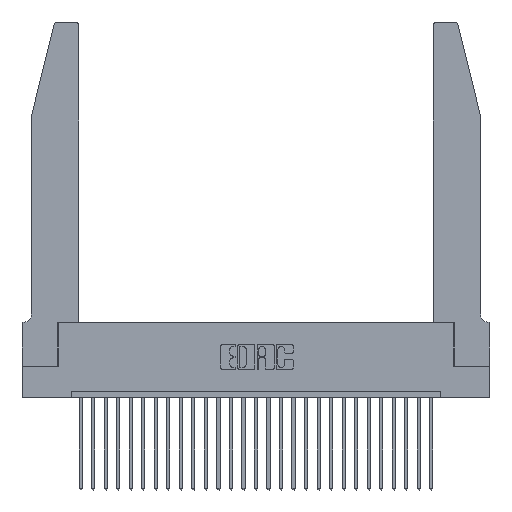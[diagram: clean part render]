
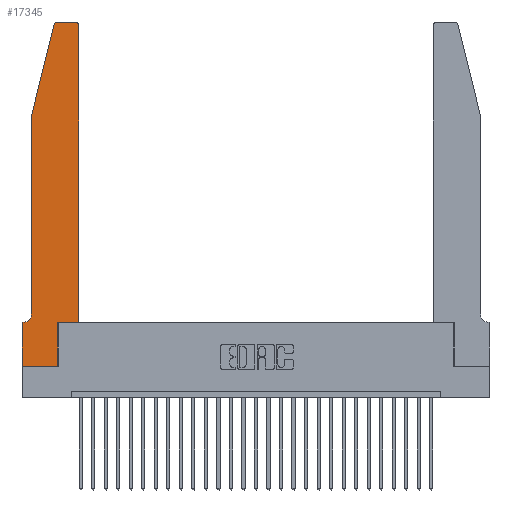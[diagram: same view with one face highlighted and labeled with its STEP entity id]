
A CAD part, top view. The second image highlights one B-rep face of the part: STEP entity #17345.
In plain terms, the highlighted planar face has unit normal (0, 0, 1).
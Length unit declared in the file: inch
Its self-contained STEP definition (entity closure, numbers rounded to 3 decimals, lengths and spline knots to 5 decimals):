
#904 = ORIENTED_EDGE ( 'NONE', *, *, #7573, .T. ) ;
#1580 = EDGE_CURVE ( 'NONE', #14980, #19679, #10628, .T. ) ;
#1957 = CARTESIAN_POINT ( 'NONE',  ( 0.284, 2.72, 0.37 ) ) ;
#2229 = LINE ( 'NONE', #5187, #10463 ) ;
#2458 = CARTESIAN_POINT ( 'NONE',  ( 0.25487, 2.72718, 0.37 ) ) ;
#2658 = CARTESIAN_POINT ( 'NONE',  ( 0., 0., 0.37 ) ) ;
#2712 = CARTESIAN_POINT ( 'NONE',  ( 0.4505, 0.35, 0.37 ) ) ;
#2842 = VERTEX_POINT ( 'NONE', #21856 ) ;
#3408 = ORIENTED_EDGE ( 'NONE', *, *, #24890, .T. ) ;
#3573 = EDGE_CURVE ( 'NONE', #14192, #27895, #18481, .T. ) ;
#3692 = ORIENTED_EDGE ( 'NONE', *, *, #3573, .T. ) ;
#4606 = VERTEX_POINT ( 'NONE', #22567 ) ;
#4884 = CIRCLE ( 'NONE', #19451, 0.07 ) ;
#5000 = ORIENTED_EDGE ( 'NONE', *, *, #16913, .T. ) ;
#5187 = CARTESIAN_POINT ( 'NONE',  ( 0.0755, 0.35, 0.37 ) ) ;
#5272 = VERTEX_POINT ( 'NONE', #11952 ) ;
#5293 = DIRECTION ( 'NONE',  ( -1., 0., 0. ) ) ;
#5399 = VERTEX_POINT ( 'NONE', #17111 ) ;
#5493 = CIRCLE ( 'NONE', #21747, 0.03 ) ;
#5974 = ORIENTED_EDGE ( 'NONE', *, *, #8012, .T. ) ;
#6187 = LINE ( 'NONE', #2658, #23042 ) ;
#6262 = DIRECTION ( 'NONE',  ( 0., 0., 1. ) ) ;
#6360 = AXIS2_PLACEMENT_3D ( 'NONE', #7596, #13937, #27242 ) ;
#6550 = ORIENTED_EDGE ( 'NONE', *, *, #9321, .T. ) ;
#6581 = EDGE_CURVE ( 'NONE', #13716, #5272, #2229, .T. ) ;
#6804 = CARTESIAN_POINT ( 'NONE',  ( 0.4505, 2.72, 0.37 ) ) ;
#7573 = EDGE_CURVE ( 'NONE', #7686, #4606, #26142, .T. ) ;
#7596 = CARTESIAN_POINT ( 'NONE',  ( 0., 0.35, 0.37 ) ) ;
#7686 = VERTEX_POINT ( 'NONE', #14139 ) ;
#8012 = EDGE_CURVE ( 'NONE', #4606, #14192, #25118, .T. ) ;
#8188 = CARTESIAN_POINT ( 'NONE',  ( 0.0755, 2., 0.37 ) ) ;
#8631 = ORIENTED_EDGE ( 'NONE', *, *, #14116, .T. ) ;
#8788 = CARTESIAN_POINT ( 'NONE',  ( 0.4205, 2.75, 0.37 ) ) ;
#9013 = VECTOR ( 'NONE', #11927, 39.37008 ) ;
#9321 = EDGE_CURVE ( 'NONE', #5399, #13716, #4884, .T. ) ;
#10112 = CARTESIAN_POINT ( 'NONE',  ( 0.2865, 0.35, 0.37 ) ) ;
#10231 = VECTOR ( 'NONE', #22392, 39.37008 ) ;
#10463 = VECTOR ( 'NONE', #5293, 39.37008 ) ;
#10628 = LINE ( 'NONE', #15338, #18875 ) ;
#11100 = DIRECTION ( 'NONE',  ( -0.239, -0.971, 0. ) ) ;
#11371 = CARTESIAN_POINT ( 'NONE',  ( 0.284, 2.75, 0.37 ) ) ;
#11375 = DIRECTION ( 'NONE',  ( 0., -1., 0. ) ) ;
#11927 = DIRECTION ( 'NONE',  ( -1., 0., 0. ) ) ;
#11952 = CARTESIAN_POINT ( 'NONE',  ( 0., 0.35, 0.37 ) ) ;
#12058 = DIRECTION ( 'NONE',  ( 0., 0., 1. ) ) ;
#12329 = DIRECTION ( 'NONE',  ( 0., 0., -1. ) ) ;
#12431 = LINE ( 'NONE', #19485, #21072 ) ;
#12522 = ORIENTED_EDGE ( 'NONE', *, *, #25599, .T. ) ;
#12996 = DIRECTION ( 'NONE',  ( 1., 0., 0. ) ) ;
#13116 = CARTESIAN_POINT ( 'NONE',  ( 0.0055, 0.35, 0.37 ) ) ;
#13120 = VECTOR ( 'NONE', #12996, 39.37008 ) ;
#13716 = VERTEX_POINT ( 'NONE', #13116 ) ;
#13937 = DIRECTION ( 'NONE',  ( 0., 0., 1. ) ) ;
#14116 = EDGE_CURVE ( 'NONE', #2842, #7686, #28347, .T. ) ;
#14139 = CARTESIAN_POINT ( 'NONE',  ( 0.2865, 0., 0.37 ) ) ;
#14192 = VERTEX_POINT ( 'NONE', #26556 ) ;
#14232 = CIRCLE ( 'NONE', #27106, 0.03 ) ;
#14272 = DIRECTION ( 'NONE',  ( 1., 0., 0. ) ) ;
#14494 = EDGE_LOOP ( 'NONE', ( #23399, #27559, #21449, #3408, #6550, #26379, #12522, #8631, #904, #5974, #3692, #5000 ) ) ;
#14980 = VERTEX_POINT ( 'NONE', #2458 ) ;
#15338 = CARTESIAN_POINT ( 'NONE',  ( 0.0755, 2., 0.37 ) ) ;
#15766 = CARTESIAN_POINT ( 'NONE',  ( 0., 0., 0.37 ) ) ;
#16856 = CARTESIAN_POINT ( 'NONE',  ( 0.4505, 0.35, 0.37 ) ) ;
#16913 = EDGE_CURVE ( 'NONE', #27895, #18076, #14232, .T. ) ;
#17111 = CARTESIAN_POINT ( 'NONE',  ( 0.0755, 0.42, 0.37 ) ) ;
#17345 = ADVANCED_FACE ( 'NONE', ( #18370 ), #18886, .T. ) ;
#17413 = VECTOR ( 'NONE', #26551, 39.37008 ) ;
#17518 = DIRECTION ( 'NONE',  ( 1., 0., 0. ) ) ;
#18076 = VERTEX_POINT ( 'NONE', #8788 ) ;
#18370 = FACE_OUTER_BOUND ( 'NONE', #14494, .T. ) ;
#18481 = LINE ( 'NONE', #2712, #17413 ) ;
#18562 = VERTEX_POINT ( 'NONE', #11371 ) ;
#18875 = VECTOR ( 'NONE', #11100, 39.37008 ) ;
#18886 = PLANE ( 'NONE',  #6360 ) ;
#19293 = EDGE_CURVE ( 'NONE', #18076, #18562, #27182, .T. ) ;
#19451 = AXIS2_PLACEMENT_3D ( 'NONE', #22994, #12329, #27623 ) ;
#19485 = CARTESIAN_POINT ( 'NONE',  ( 0.0755, 2., 0.37 ) ) ;
#19679 = VERTEX_POINT ( 'NONE', #8188 ) ;
#21072 = VECTOR ( 'NONE', #26139, 39.37008 ) ;
#21449 = ORIENTED_EDGE ( 'NONE', *, *, #1580, .T. ) ;
#21735 = VECTOR ( 'NONE', #25257, 39.37008 ) ;
#21747 = AXIS2_PLACEMENT_3D ( 'NONE', #1957, #6262, #17518 ) ;
#21856 = CARTESIAN_POINT ( 'NONE',  ( 0., 0., 0.37 ) ) ;
#22109 = EDGE_CURVE ( 'NONE', #18562, #14980, #5493, .T. ) ;
#22392 = DIRECTION ( 'NONE',  ( 1., 0., 0. ) ) ;
#22567 = CARTESIAN_POINT ( 'NONE',  ( 0.2865, 0.35, 0.37 ) ) ;
#22994 = CARTESIAN_POINT ( 'NONE',  ( 0.0055, 0.42, 0.37 ) ) ;
#23042 = VECTOR ( 'NONE', #11375, 39.37008 ) ;
#23399 = ORIENTED_EDGE ( 'NONE', *, *, #19293, .T. ) ;
#24890 = EDGE_CURVE ( 'NONE', #19679, #5399, #12431, .T. ) ;
#25118 = LINE ( 'NONE', #16856, #13120 ) ;
#25133 = CARTESIAN_POINT ( 'NONE',  ( 0.2605, 2.75, 0.37 ) ) ;
#25257 = DIRECTION ( 'NONE',  ( 0., 1., 0. ) ) ;
#25346 = CARTESIAN_POINT ( 'NONE',  ( 0.4205, 2.72, 0.37 ) ) ;
#25599 = EDGE_CURVE ( 'NONE', #5272, #2842, #6187, .T. ) ;
#26139 = DIRECTION ( 'NONE',  ( 0., -1., 0. ) ) ;
#26142 = LINE ( 'NONE', #10112, #21735 ) ;
#26379 = ORIENTED_EDGE ( 'NONE', *, *, #6581, .T. ) ;
#26551 = DIRECTION ( 'NONE',  ( 0., 1., 0. ) ) ;
#26556 = CARTESIAN_POINT ( 'NONE',  ( 0.4505, 0.35, 0.37 ) ) ;
#27106 = AXIS2_PLACEMENT_3D ( 'NONE', #25346, #12058, #14272 ) ;
#27182 = LINE ( 'NONE', #25133, #9013 ) ;
#27242 = DIRECTION ( 'NONE',  ( 1., 0., 0. ) ) ;
#27559 = ORIENTED_EDGE ( 'NONE', *, *, #22109, .T. ) ;
#27623 = DIRECTION ( 'NONE',  ( -1., 0., 0. ) ) ;
#27895 = VERTEX_POINT ( 'NONE', #6804 ) ;
#28347 = LINE ( 'NONE', #15766, #10231 ) ;
